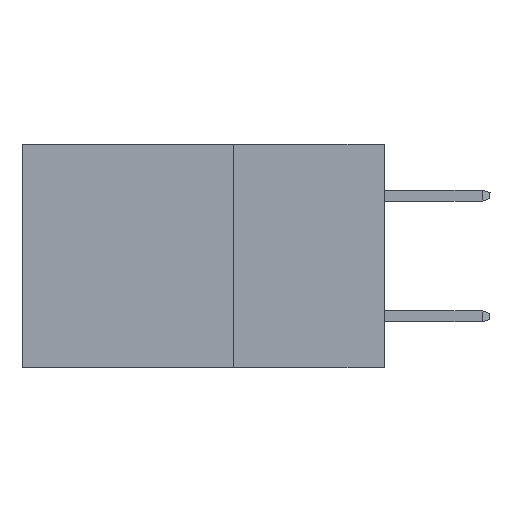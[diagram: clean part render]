
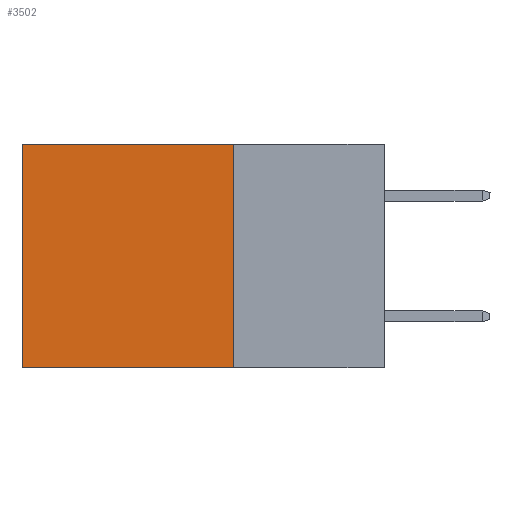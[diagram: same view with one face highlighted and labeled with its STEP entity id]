
A CAD part, left-side view. The second image highlights one B-rep face of the part: STEP entity #3502.
In plain terms, the highlighted planar face has unit normal (-1, 0, 0).
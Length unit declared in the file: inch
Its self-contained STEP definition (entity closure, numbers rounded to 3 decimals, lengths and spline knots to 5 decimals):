
#311 = EDGE_CURVE ( 'NONE', #8794, #9738, #27434, .T. ) ;
#3102 = DIRECTION ( 'NONE',  ( 0., 0., -1. ) ) ;
#3502 = ADVANCED_FACE ( 'NONE', ( #7995 ), #23768, .F. ) ;
#3773 = LINE ( 'NONE', #4187, #12027 ) ;
#4187 = CARTESIAN_POINT ( 'NONE',  ( 0.298, 0.6, 0. ) ) ;
#4294 = DIRECTION ( 'NONE',  ( 0., 0., -1. ) ) ;
#4936 = LINE ( 'NONE', #16006, #8495 ) ;
#5153 = ORIENTED_EDGE ( 'NONE', *, *, #25583, .T. ) ;
#5367 = ORIENTED_EDGE ( 'NONE', *, *, #23088, .T. ) ;
#7995 = FACE_OUTER_BOUND ( 'NONE', #17686, .T. ) ;
#8495 = VECTOR ( 'NONE', #23713, 39.37008 ) ;
#8794 = VERTEX_POINT ( 'NONE', #19335 ) ;
#9738 = VERTEX_POINT ( 'NONE', #20210 ) ;
#10467 = CARTESIAN_POINT ( 'NONE',  ( 0.298, 0.6, -0.37 ) ) ;
#12027 = VECTOR ( 'NONE', #4294, 39.37008 ) ;
#15630 = CARTESIAN_POINT ( 'NONE',  ( 0.298, 0.25, 0. ) ) ;
#16006 = CARTESIAN_POINT ( 'NONE',  ( 0.298, 0.25, -0.37 ) ) ;
#17686 = EDGE_LOOP ( 'NONE', ( #5153, #24277, #19592, #5367 ) ) ;
#18711 = DIRECTION ( 'NONE',  ( 0., 0., -1. ) ) ;
#19247 = VERTEX_POINT ( 'NONE', #28697 ) ;
#19335 = CARTESIAN_POINT ( 'NONE',  ( 0.298, 0.25, 0. ) ) ;
#19592 = ORIENTED_EDGE ( 'NONE', *, *, #311, .F. ) ;
#20210 = CARTESIAN_POINT ( 'NONE',  ( 0.298, 0.25, -0.37 ) ) ;
#20814 = CARTESIAN_POINT ( 'NONE',  ( 0.298, 0.25, 0. ) ) ;
#23088 = EDGE_CURVE ( 'NONE', #8794, #19247, #32165, .T. ) ;
#23685 = AXIS2_PLACEMENT_3D ( 'NONE', #26525, #31606, #18711 ) ;
#23713 = DIRECTION ( 'NONE',  ( 0., 1., 0. ) ) ;
#23768 = PLANE ( 'NONE',  #23685 ) ;
#24277 = ORIENTED_EDGE ( 'NONE', *, *, #25853, .F. ) ;
#25057 = VECTOR ( 'NONE', #3102, 39.37008 ) ;
#25436 = DIRECTION ( 'NONE',  ( 0., 1., 0. ) ) ;
#25449 = VECTOR ( 'NONE', #25436, 39.37008 ) ;
#25583 = EDGE_CURVE ( 'NONE', #19247, #29401, #3773, .T. ) ;
#25853 = EDGE_CURVE ( 'NONE', #9738, #29401, #4936, .T. ) ;
#26525 = CARTESIAN_POINT ( 'NONE',  ( 0.298, 0.25, 0. ) ) ;
#27434 = LINE ( 'NONE', #15630, #25057 ) ;
#28697 = CARTESIAN_POINT ( 'NONE',  ( 0.298, 0.6, 0. ) ) ;
#29401 = VERTEX_POINT ( 'NONE', #10467 ) ;
#31606 = DIRECTION ( 'NONE',  ( 1., 0., 0. ) ) ;
#32165 = LINE ( 'NONE', #20814, #25449 ) ;
